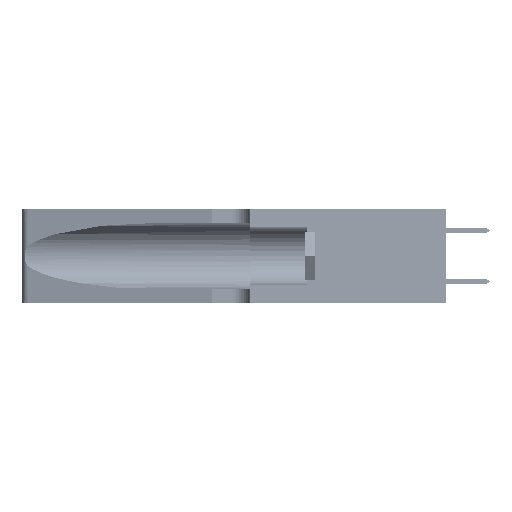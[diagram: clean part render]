
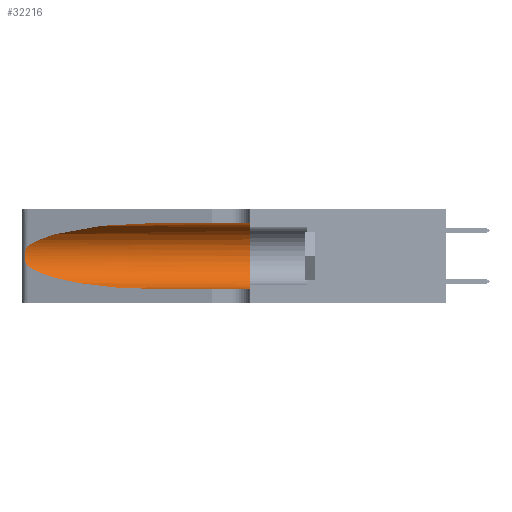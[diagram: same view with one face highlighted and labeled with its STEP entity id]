
A CAD part, left-side view. The second image highlights one B-rep face of the part: STEP entity #32216.
In plain terms, the highlighted cylindrical face has radius 3.308 mm (diameter 6.617 mm), a partial arc.
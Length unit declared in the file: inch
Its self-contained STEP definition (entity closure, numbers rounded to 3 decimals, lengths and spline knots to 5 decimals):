
#159 = ORIENTED_EDGE ( 'NONE', *, *, #33255, .T. ) ;
#1399 = CARTESIAN_POINT ( 'NONE',  ( 0.25789, 1.23486, 0.15765 ) ) ;
#1697 = CARTESIAN_POINT ( 'NONE',  ( 0.1305, 0.35, 0.31525 ) ) ;
#1946 = CARTESIAN_POINT ( 'NONE',  ( 0.25854, 1.2359, 0.20912 ) ) ;
#5861 = CARTESIAN_POINT ( 'NONE',  ( 0.25487, 1.22718, 0.14631 ) ) ;
#7720 = EDGE_CURVE ( 'NONE', #35975, #54162, #39250, .T. ) ;
#8455 = EDGE_CURVE ( 'NONE', #43814, #39954, #26194, .T. ) ;
#9923 = CARTESIAN_POINT ( 'NONE',  ( 0.26075, 1.23896, 0.178 ) ) ;
#9964 = CARTESIAN_POINT ( 'NONE',  ( 0.25487, 1.22718, 0.22369 ) ) ;
#13487 = VERTEX_POINT ( 'NONE', #44285 ) ;
#15589 = CARTESIAN_POINT ( 'NONE',  ( 0.1305, 0.72297, 0.05475 ) ) ;
#16203 = CARTESIAN_POINT ( 'NONE',  ( 0.1305, 1.61858, 0.05475 ) ) ;
#17456 = CARTESIAN_POINT ( 'NONE',  ( 0.1305, 0.72297, 0.05475 ) ) ;
#18223 = CARTESIAN_POINT ( 'NONE',  ( 0.25487, 1.22718, 0.22369 ) ) ;
#19781 = EDGE_LOOP ( 'NONE', ( #159, #28078, #52231, #34384, #49561, #33600 ) ) ;
#21560 = DIRECTION ( 'NONE',  ( 0., -1., 0. ) ) ;
#21858 = LINE ( 'NONE', #32864, #44498 ) ;
#22659 = CARTESIAN_POINT ( 'NONE',  ( 0.26017, 1.23833, 0.17102 ) ) ;
#23025 = CARTESIAN_POINT ( 'NONE',  ( 0.26075, 1.23896, 0.19203 ) ) ;
#24614 = EDGE_CURVE ( 'NONE', #54162, #39954, #30775, .T. ) ;
#25556 =( BOUNDED_CURVE ( )  B_SPLINE_CURVE ( 3, ( #47799, #31120, #40032, #9964 ),
 .UNSPECIFIED., .F., .T. ) 
 B_SPLINE_CURVE_WITH_KNOTS ( ( 4, 4 ),
 ( 1.5708, 2.84003 ),
 .UNSPECIFIED. ) 
 CURVE ( )  GEOMETRIC_REPRESENTATION_ITEM ( )  RATIONAL_B_SPLINE_CURVE ( ( 1., 0.87, 0.87, 1. ) ) 
 REPRESENTATION_ITEM ( '' )  );
#25656 = CARTESIAN_POINT ( 'NONE',  ( 0.2373, 1.15595, 0.08982 ) ) ;
#26194 = CIRCLE ( 'NONE', #26367, 0.13025 ) ;
#26367 = AXIS2_PLACEMENT_3D ( 'NONE', #43626, #31191, #39188 ) ;
#26782 = CARTESIAN_POINT ( 'NONE',  ( 0.25639, 1.23186, 0.15144 ) ) ;
#28078 = ORIENTED_EDGE ( 'NONE', *, *, #33814, .T. ) ;
#28514 = EDGE_CURVE ( 'NONE', #47025, #43814, #21858, .T. ) ;
#29533 = CARTESIAN_POINT ( 'NONE',  ( 0.1305, 1.61858, 0.185 ) ) ;
#30775 = LINE ( 'NONE', #16203, #47374 ) ;
#31120 = CARTESIAN_POINT ( 'NONE',  ( 0.18966, 0.96281, 0.31525 ) ) ;
#31191 = DIRECTION ( 'NONE',  ( 0., 1., 0. ) ) ;
#32216 = ADVANCED_FACE ( 'NONE', ( #39489 ), #34177, .F. ) ;
#32864 = CARTESIAN_POINT ( 'NONE',  ( 0.1305, 1.61858, 0.31525 ) ) ;
#33082 = DIRECTION ( 'NONE',  ( 0., -1., 0. ) ) ;
#33255 = EDGE_CURVE ( 'NONE', #47025, #13487, #25556, .T. ) ;
#33600 = ORIENTED_EDGE ( 'NONE', *, *, #28514, .F. ) ;
#33814 = EDGE_CURVE ( 'NONE', #13487, #35975, #47017, .T. ) ;
#34177 = CYLINDRICAL_SURFACE ( 'NONE', #48404, 0.13025 ) ;
#34384 = ORIENTED_EDGE ( 'NONE', *, *, #24614, .T. ) ;
#35570 = CARTESIAN_POINT ( 'NONE',  ( 0.25639, 1.23184, 0.21858 ) ) ;
#35975 = VERTEX_POINT ( 'NONE', #41250 ) ;
#38534 = CARTESIAN_POINT ( 'NONE',  ( 0.25487, 1.22718, 0.14631 ) ) ;
#39188 = DIRECTION ( 'NONE',  ( 0., 0., 1. ) ) ;
#39250 =( BOUNDED_CURVE ( )  B_SPLINE_CURVE ( 3, ( #38534, #25656, #46835, #17456 ),
 .UNSPECIFIED., .F., .T. ) 
 B_SPLINE_CURVE_WITH_KNOTS ( ( 4, 4 ),
 ( 3.44316, 4.71239 ),
 .UNSPECIFIED. ) 
 CURVE ( )  GEOMETRIC_REPRESENTATION_ITEM ( )  RATIONAL_B_SPLINE_CURVE ( ( 1., 0.87, 0.87, 1. ) ) 
 REPRESENTATION_ITEM ( '' )  );
#39489 = FACE_OUTER_BOUND ( 'NONE', #19781, .T. ) ;
#39813 = CARTESIAN_POINT ( 'NONE',  ( 0.25856, 1.23593, 0.16098 ) ) ;
#39954 = VERTEX_POINT ( 'NONE', #47423 ) ;
#40032 = CARTESIAN_POINT ( 'NONE',  ( 0.2373, 1.15595, 0.28018 ) ) ;
#40746 = CARTESIAN_POINT ( 'NONE',  ( 0.1305, 0.72297, 0.31525 ) ) ;
#41250 = CARTESIAN_POINT ( 'NONE',  ( 0.25487, 1.22718, 0.14631 ) ) ;
#43626 = CARTESIAN_POINT ( 'NONE',  ( 0.1305, 0.35, 0.185 ) ) ;
#43814 = VERTEX_POINT ( 'NONE', #1697 ) ;
#44285 = CARTESIAN_POINT ( 'NONE',  ( 0.25487, 1.22718, 0.22369 ) ) ;
#44413 = CARTESIAN_POINT ( 'NONE',  ( 0.26018, 1.23835, 0.19895 ) ) ;
#44498 = VECTOR ( 'NONE', #49532, 39.37008 ) ;
#46835 = CARTESIAN_POINT ( 'NONE',  ( 0.18966, 0.96281, 0.05475 ) ) ;
#47017 = B_SPLINE_CURVE_WITH_KNOTS ( 'NONE', 3,
 ( #18223, #47934, #35570, #48125, #1946, #44413, #23025, #9923, #22659, #39813, #1399, #26782, #52385, #5861 ),
 .UNSPECIFIED., .F., .F.,
 ( 4, 2, 2, 2, 2, 2, 4 ),
 ( 0., 0.00027, 0.00053, 0.00107, 0.0016, 0.00187, 0.00214 ),
 .UNSPECIFIED. ) ;
#47025 = VERTEX_POINT ( 'NONE', #40746 ) ;
#47374 = VECTOR ( 'NONE', #21560, 39.37008 ) ;
#47423 = CARTESIAN_POINT ( 'NONE',  ( 0.1305, 0.35, 0.05475 ) ) ;
#47799 = CARTESIAN_POINT ( 'NONE',  ( 0.1305, 0.72297, 0.31525 ) ) ;
#47934 = CARTESIAN_POINT ( 'NONE',  ( 0.25555, 1.22994, 0.2215 ) ) ;
#48125 = CARTESIAN_POINT ( 'NONE',  ( 0.25787, 1.23484, 0.2124 ) ) ;
#48404 = AXIS2_PLACEMENT_3D ( 'NONE', #29533, #33082, #50668 ) ;
#49532 = DIRECTION ( 'NONE',  ( 0., -1., 0. ) ) ;
#49561 = ORIENTED_EDGE ( 'NONE', *, *, #8455, .F. ) ;
#50668 = DIRECTION ( 'NONE',  ( 0., 0., -1. ) ) ;
#52231 = ORIENTED_EDGE ( 'NONE', *, *, #7720, .T. ) ;
#52385 = CARTESIAN_POINT ( 'NONE',  ( 0.25555, 1.22993, 0.14849 ) ) ;
#54162 = VERTEX_POINT ( 'NONE', #15589 ) ;
